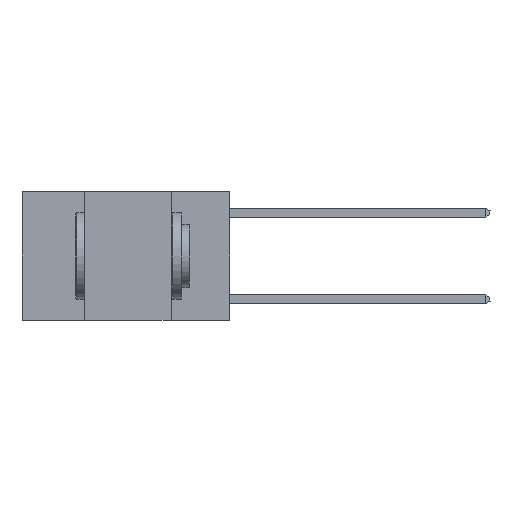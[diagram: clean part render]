
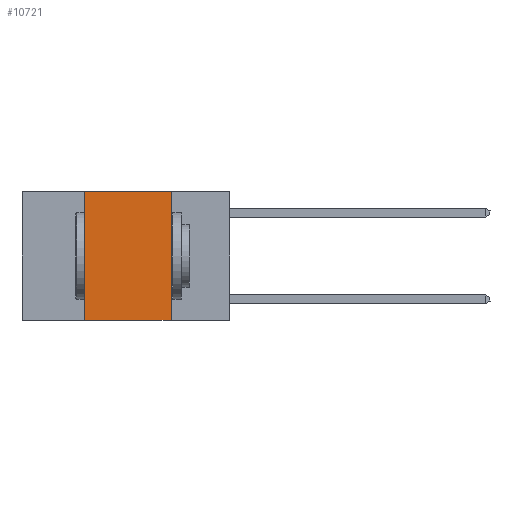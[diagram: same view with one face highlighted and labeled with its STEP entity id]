
A CAD part, left-side view. The second image highlights one B-rep face of the part: STEP entity #10721.
In plain terms, the highlighted planar face has unit normal (-1, 0, 0).
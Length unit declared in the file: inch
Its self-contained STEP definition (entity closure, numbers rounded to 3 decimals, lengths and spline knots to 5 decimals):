
#1622 = CARTESIAN_POINT ( 'NONE',  ( 0., 0.6, 0. ) ) ;
#2057 = EDGE_CURVE ( 'NONE', #3378, #22143, #9517, .T. ) ;
#3378 = VERTEX_POINT ( 'NONE', #26344 ) ;
#3720 = CARTESIAN_POINT ( 'NONE',  ( 0., 0.17, 0. ) ) ;
#3776 = DIRECTION ( 'NONE',  ( 0., -1., 0. ) ) ;
#5390 = LINE ( 'NONE', #12019, #31140 ) ;
#6314 = CARTESIAN_POINT ( 'NONE',  ( 0., 0.6, 0. ) ) ;
#6699 = DIRECTION ( 'NONE',  ( 1., 0., 0. ) ) ;
#7023 = DIRECTION ( 'NONE',  ( 0., 0., 1. ) ) ;
#7206 = EDGE_CURVE ( 'NONE', #16675, #3378, #5390, .T. ) ;
#7869 = DIRECTION ( 'NONE',  ( 0., -1., 0. ) ) ;
#9517 = LINE ( 'NONE', #6314, #21247 ) ;
#10721 = ADVANCED_FACE ( 'NONE', ( #11739 ), #26584, .F. ) ;
#11739 = FACE_OUTER_BOUND ( 'NONE', #17121, .T. ) ;
#12019 = CARTESIAN_POINT ( 'NONE',  ( 0., 0.42, 0. ) ) ;
#12169 = VECTOR ( 'NONE', #7869, 39.37008 ) ;
#12725 = EDGE_CURVE ( 'NONE', #22143, #30437, #26802, .T. ) ;
#15401 = ORIENTED_EDGE ( 'NONE', *, *, #7206, .F. ) ;
#16183 = ORIENTED_EDGE ( 'NONE', *, *, #27051, .T. ) ;
#16675 = VERTEX_POINT ( 'NONE', #28974 ) ;
#17026 = CARTESIAN_POINT ( 'NONE',  ( 0., 0.17, 0. ) ) ;
#17121 = EDGE_LOOP ( 'NONE', ( #32067, #19665, #15401, #16183 ) ) ;
#19665 = ORIENTED_EDGE ( 'NONE', *, *, #2057, .F. ) ;
#20204 = VECTOR ( 'NONE', #27014, 39.37008 ) ;
#21247 = VECTOR ( 'NONE', #3776, 39.37008 ) ;
#22143 = VERTEX_POINT ( 'NONE', #3720 ) ;
#23087 = CARTESIAN_POINT ( 'NONE',  ( 0., 0.17, -0.37 ) ) ;
#24230 = DIRECTION ( 'NONE',  ( 0., 0., -1. ) ) ;
#25386 = LINE ( 'NONE', #27805, #12169 ) ;
#26344 = CARTESIAN_POINT ( 'NONE',  ( 0., 0.42, 0. ) ) ;
#26552 = AXIS2_PLACEMENT_3D ( 'NONE', #1622, #6699, #24230 ) ;
#26584 = PLANE ( 'NONE',  #26552 ) ;
#26802 = LINE ( 'NONE', #17026, #20204 ) ;
#27014 = DIRECTION ( 'NONE',  ( 0., 0., -1. ) ) ;
#27051 = EDGE_CURVE ( 'NONE', #16675, #30437, #25386, .T. ) ;
#27805 = CARTESIAN_POINT ( 'NONE',  ( 0., 0.6, -0.37 ) ) ;
#28974 = CARTESIAN_POINT ( 'NONE',  ( 0., 0.42, -0.37 ) ) ;
#30437 = VERTEX_POINT ( 'NONE', #23087 ) ;
#31140 = VECTOR ( 'NONE', #7023, 39.37008 ) ;
#32067 = ORIENTED_EDGE ( 'NONE', *, *, #12725, .F. ) ;
